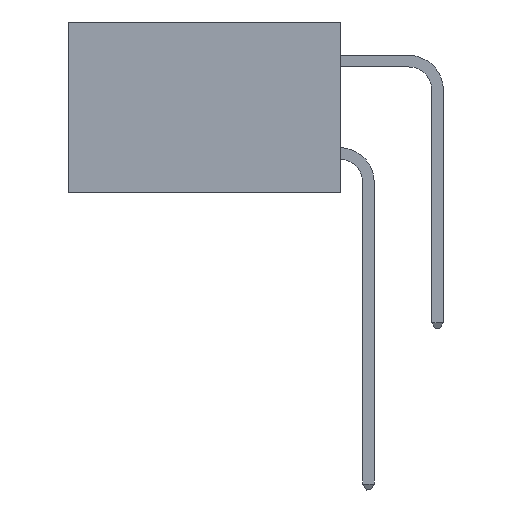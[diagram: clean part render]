
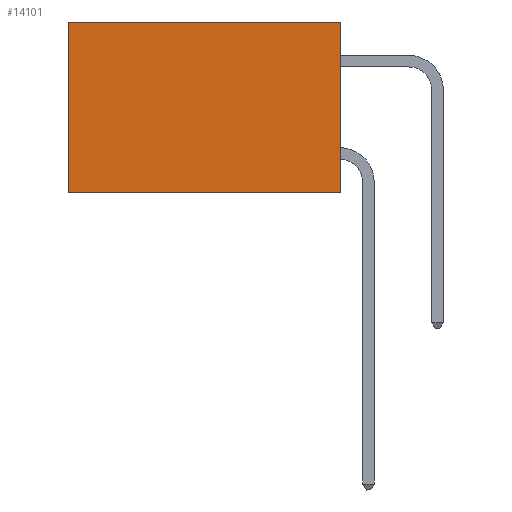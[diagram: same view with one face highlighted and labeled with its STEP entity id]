
A CAD part, left-side view. The second image highlights one B-rep face of the part: STEP entity #14101.
In plain terms, the highlighted planar face has unit normal (-1, 0, 0).
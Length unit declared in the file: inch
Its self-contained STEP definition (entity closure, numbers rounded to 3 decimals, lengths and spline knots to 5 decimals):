
#1262 = DIRECTION ( 'NONE',  ( 0., 0., -1. ) ) ;
#1348 = CARTESIAN_POINT ( 'NONE',  ( 0.277, 0., -0.37 ) ) ;
#1741 = DIRECTION ( 'NONE',  ( 0., 1., 0. ) ) ;
#1917 = VERTEX_POINT ( 'NONE', #17398 ) ;
#2071 = ORIENTED_EDGE ( 'NONE', *, *, #5775, .F. ) ;
#2186 = LINE ( 'NONE', #7134, #15150 ) ;
#4188 = VERTEX_POINT ( 'NONE', #20210 ) ;
#4526 = ORIENTED_EDGE ( 'NONE', *, *, #22733, .T. ) ;
#5775 = EDGE_CURVE ( 'NONE', #9140, #4188, #23981, .T. ) ;
#7134 = CARTESIAN_POINT ( 'NONE',  ( 0.277, 0.59, -0.37 ) ) ;
#9140 = VERTEX_POINT ( 'NONE', #20674 ) ;
#9532 = EDGE_LOOP ( 'NONE', ( #24572, #2071, #32875, #4526 ) ) ;
#9649 = FACE_OUTER_BOUND ( 'NONE', #9532, .T. ) ;
#9706 = LINE ( 'NONE', #29489, #22671 ) ;
#11012 = EDGE_CURVE ( 'NONE', #1917, #4188, #2186, .T. ) ;
#11289 = AXIS2_PLACEMENT_3D ( 'NONE', #21895, #16807, #1262 ) ;
#13104 = CARTESIAN_POINT ( 'NONE',  ( 0.277, 0., 0. ) ) ;
#13916 = DIRECTION ( 'NONE',  ( 0., 1., 0. ) ) ;
#14101 = ADVANCED_FACE ( 'NONE', ( #9649 ), #29732, .F. ) ;
#14945 = DIRECTION ( 'NONE',  ( 0., 0., -1. ) ) ;
#15150 = VECTOR ( 'NONE', #14945, 39.37008 ) ;
#15647 = DIRECTION ( 'NONE',  ( 0., 0., -1. ) ) ;
#16807 = DIRECTION ( 'NONE',  ( 1., 0., 0. ) ) ;
#17398 = CARTESIAN_POINT ( 'NONE',  ( 0.277, 0.59, 0. ) ) ;
#18514 = EDGE_CURVE ( 'NONE', #20889, #9140, #27352, .T. ) ;
#20210 = CARTESIAN_POINT ( 'NONE',  ( 0.277, 0.59, -0.37 ) ) ;
#20674 = CARTESIAN_POINT ( 'NONE',  ( 0.277, 0., -0.37 ) ) ;
#20889 = VERTEX_POINT ( 'NONE', #13104 ) ;
#21895 = CARTESIAN_POINT ( 'NONE',  ( 0.277, 0., -0.37 ) ) ;
#22671 = VECTOR ( 'NONE', #13916, 39.37008 ) ;
#22733 = EDGE_CURVE ( 'NONE', #20889, #1917, #9706, .T. ) ;
#23183 = VECTOR ( 'NONE', #1741, 39.37008 ) ;
#23981 = LINE ( 'NONE', #1348, #23183 ) ;
#24572 = ORIENTED_EDGE ( 'NONE', *, *, #11012, .T. ) ;
#27352 = LINE ( 'NONE', #31052, #31785 ) ;
#29489 = CARTESIAN_POINT ( 'NONE',  ( 0.277, 0., 0. ) ) ;
#29732 = PLANE ( 'NONE',  #11289 ) ;
#31052 = CARTESIAN_POINT ( 'NONE',  ( 0.277, 0., -0.37 ) ) ;
#31785 = VECTOR ( 'NONE', #15647, 39.37008 ) ;
#32875 = ORIENTED_EDGE ( 'NONE', *, *, #18514, .F. ) ;
